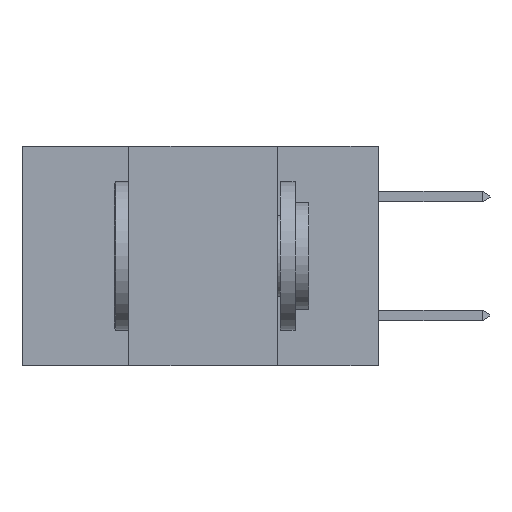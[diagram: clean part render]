
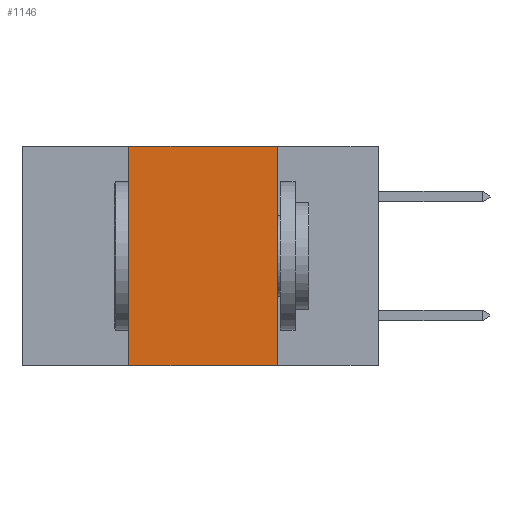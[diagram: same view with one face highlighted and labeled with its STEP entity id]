
A CAD part, left-side view. The second image highlights one B-rep face of the part: STEP entity #1146.
In plain terms, the highlighted planar face has unit normal (-1, 0, 0).
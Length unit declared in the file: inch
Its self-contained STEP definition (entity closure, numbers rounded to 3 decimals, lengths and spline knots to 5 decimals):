
#372 = LINE ( 'NONE', #1071, #12070 ) ;
#1071 = CARTESIAN_POINT ( 'NONE',  ( 0., 0.6, -0.37 ) ) ;
#1146 = ADVANCED_FACE ( 'NONE', ( #16350 ), #16519, .F. ) ;
#1901 = CARTESIAN_POINT ( 'NONE',  ( 0., 0.17, 0. ) ) ;
#2030 = VERTEX_POINT ( 'NONE', #1901 ) ;
#2456 = EDGE_LOOP ( 'NONE', ( #5421, #12880, #15406, #6867 ) ) ;
#2895 = LINE ( 'NONE', #11157, #4411 ) ;
#3489 = CARTESIAN_POINT ( 'NONE',  ( 0., 0.17, 0. ) ) ;
#3745 = CARTESIAN_POINT ( 'NONE',  ( 0., 0.42, 0. ) ) ;
#4118 = VERTEX_POINT ( 'NONE', #5839 ) ;
#4281 = CARTESIAN_POINT ( 'NONE',  ( 0., 0.42, 0. ) ) ;
#4411 = VECTOR ( 'NONE', #11382, 39.37008 ) ;
#4657 = VERTEX_POINT ( 'NONE', #6870 ) ;
#5421 = ORIENTED_EDGE ( 'NONE', *, *, #5581, .F. ) ;
#5581 = EDGE_CURVE ( 'NONE', #2030, #4657, #11211, .T. ) ;
#5839 = CARTESIAN_POINT ( 'NONE',  ( 0., 0.42, -0.37 ) ) ;
#5863 = EDGE_CURVE ( 'NONE', #4118, #4657, #372, .T. ) ;
#6867 = ORIENTED_EDGE ( 'NONE', *, *, #5863, .T. ) ;
#6870 = CARTESIAN_POINT ( 'NONE',  ( 0., 0.17, -0.37 ) ) ;
#7999 = DIRECTION ( 'NONE',  ( 0., 0., -1. ) ) ;
#8168 = VERTEX_POINT ( 'NONE', #4281 ) ;
#9742 = AXIS2_PLACEMENT_3D ( 'NONE', #14837, #14961, #7999 ) ;
#9823 = EDGE_CURVE ( 'NONE', #4118, #8168, #11685, .T. ) ;
#9962 = VECTOR ( 'NONE', #13525, 39.37008 ) ;
#10346 = DIRECTION ( 'NONE',  ( 0., 0., -1. ) ) ;
#10779 = DIRECTION ( 'NONE',  ( 0., -1., 0. ) ) ;
#11157 = CARTESIAN_POINT ( 'NONE',  ( 0., 0.6, 0. ) ) ;
#11211 = LINE ( 'NONE', #3489, #14041 ) ;
#11382 = DIRECTION ( 'NONE',  ( 0., -1., 0. ) ) ;
#11685 = LINE ( 'NONE', #3745, #9962 ) ;
#12070 = VECTOR ( 'NONE', #10779, 39.37008 ) ;
#12880 = ORIENTED_EDGE ( 'NONE', *, *, #13631, .F. ) ;
#13525 = DIRECTION ( 'NONE',  ( 0., 0., 1. ) ) ;
#13631 = EDGE_CURVE ( 'NONE', #8168, #2030, #2895, .T. ) ;
#14041 = VECTOR ( 'NONE', #10346, 39.37008 ) ;
#14837 = CARTESIAN_POINT ( 'NONE',  ( 0., 0.6, 0. ) ) ;
#14961 = DIRECTION ( 'NONE',  ( 1., 0., 0. ) ) ;
#15406 = ORIENTED_EDGE ( 'NONE', *, *, #9823, .F. ) ;
#16350 = FACE_OUTER_BOUND ( 'NONE', #2456, .T. ) ;
#16519 = PLANE ( 'NONE',  #9742 ) ;
